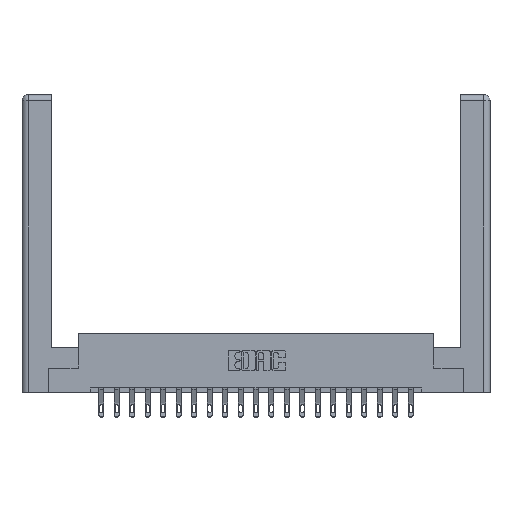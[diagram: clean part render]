
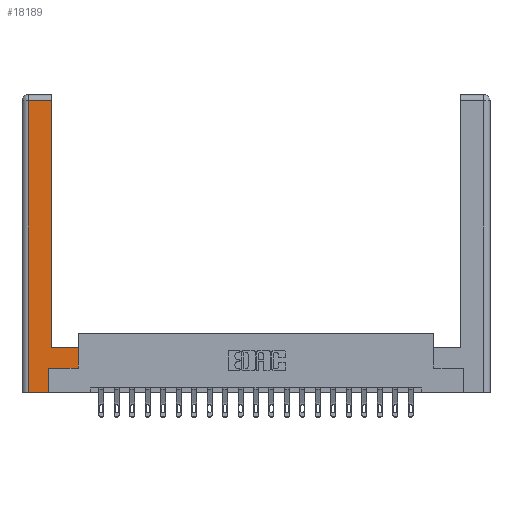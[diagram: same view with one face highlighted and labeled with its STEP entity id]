
A CAD part, top view. The second image highlights one B-rep face of the part: STEP entity #18189.
In plain terms, the highlighted planar face has unit normal (0, 0, 1).
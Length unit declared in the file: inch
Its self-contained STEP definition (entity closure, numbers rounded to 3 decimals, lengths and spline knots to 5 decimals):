
#303 = EDGE_CURVE ( 'NONE', #4934, #14037, #21726, .T. ) ;
#592 = VERTEX_POINT ( 'NONE', #5623 ) ;
#604 = DIRECTION ( 'NONE',  ( 1., 0., 0. ) ) ;
#1045 = CARTESIAN_POINT ( 'NONE',  ( 0.0615, 0., 0. ) ) ;
#1606 = DIRECTION ( 'NONE',  ( 1., 0., 0. ) ) ;
#1662 = LINE ( 'NONE', #15272, #3264 ) ;
#2182 = VECTOR ( 'NONE', #604, 39.37008 ) ;
#2737 = DIRECTION ( 'NONE',  ( -1., 0., 0. ) ) ;
#2754 = ORIENTED_EDGE ( 'NONE', *, *, #4813, .T. ) ;
#2914 = EDGE_LOOP ( 'NONE', ( #16398, #19296, #11142, #20492, #2754, #13698, #19203, #19072 ) ) ;
#3264 = VECTOR ( 'NONE', #1606, 39.37008 ) ;
#3643 = DIRECTION ( 'NONE',  ( 0., 1., 0. ) ) ;
#3861 = LINE ( 'NONE', #11119, #15807 ) ;
#4012 = LINE ( 'NONE', #9104, #15720 ) ;
#4514 = CARTESIAN_POINT ( 'NONE',  ( 0.565, 0.45, 0. ) ) ;
#4813 = EDGE_CURVE ( 'NONE', #12583, #592, #6343, .T. ) ;
#4861 = CARTESIAN_POINT ( 'NONE',  ( 0.265, 0., 0. ) ) ;
#4934 = VERTEX_POINT ( 'NONE', #6901 ) ;
#5126 = DIRECTION ( 'NONE',  ( 0., 0., -1. ) ) ;
#5623 = CARTESIAN_POINT ( 'NONE',  ( 0.265, 0.245, 0. ) ) ;
#5866 = CARTESIAN_POINT ( 'NONE',  ( 0.0615, 0., 0. ) ) ;
#5946 = DIRECTION ( 'NONE',  ( 0., -1., 0. ) ) ;
#6016 = CARTESIAN_POINT ( 'NONE',  ( 0.295, 2.94, 0. ) ) ;
#6152 = EDGE_CURVE ( 'NONE', #15660, #20231, #3861, .T. ) ;
#6343 = LINE ( 'NONE', #16733, #9555 ) ;
#6764 = CARTESIAN_POINT ( 'NONE',  ( 0., 0., 0. ) ) ;
#6901 = CARTESIAN_POINT ( 'NONE',  ( 0.0615, 2.94, 0. ) ) ;
#7133 = CARTESIAN_POINT ( 'NONE',  ( 0.295, 3., 0. ) ) ;
#7845 = LINE ( 'NONE', #7133, #21127 ) ;
#8257 = EDGE_CURVE ( 'NONE', #592, #13716, #12026, .T. ) ;
#9019 = CARTESIAN_POINT ( 'NONE',  ( 0.565, 0.245, 0. ) ) ;
#9048 = EDGE_CURVE ( 'NONE', #20231, #12795, #7845, .T. ) ;
#9104 = CARTESIAN_POINT ( 'NONE',  ( 0.0615, 2.94, 0. ) ) ;
#9362 = VECTOR ( 'NONE', #16579, 39.37008 ) ;
#9555 = VECTOR ( 'NONE', #11904, 39.37008 ) ;
#9833 = CARTESIAN_POINT ( 'NONE',  ( 0.565, 0.45, 0. ) ) ;
#10661 = DIRECTION ( 'NONE',  ( -1., 0., 0. ) ) ;
#11119 = CARTESIAN_POINT ( 'NONE',  ( 0.295, 0.45, 0. ) ) ;
#11142 = ORIENTED_EDGE ( 'NONE', *, *, #303, .T. ) ;
#11904 = DIRECTION ( 'NONE',  ( 0., 1., 0. ) ) ;
#12026 = LINE ( 'NONE', #9019, #2182 ) ;
#12583 = VERTEX_POINT ( 'NONE', #4861 ) ;
#12795 = VERTEX_POINT ( 'NONE', #6016 ) ;
#13532 = PLANE ( 'NONE',  #14444 ) ;
#13646 = EDGE_CURVE ( 'NONE', #14037, #12583, #1662, .T. ) ;
#13698 = ORIENTED_EDGE ( 'NONE', *, *, #8257, .T. ) ;
#13716 = VERTEX_POINT ( 'NONE', #18994 ) ;
#13880 = LINE ( 'NONE', #9833, #9362 ) ;
#14037 = VERTEX_POINT ( 'NONE', #1045 ) ;
#14373 = CARTESIAN_POINT ( 'NONE',  ( 0.295, 0.45, 0. ) ) ;
#14444 = AXIS2_PLACEMENT_3D ( 'NONE', #6764, #5126, #20420 ) ;
#14504 = EDGE_CURVE ( 'NONE', #13716, #15660, #13880, .T. ) ;
#14823 = VECTOR ( 'NONE', #5946, 39.37008 ) ;
#15272 = CARTESIAN_POINT ( 'NONE',  ( 0.265, 0., 0. ) ) ;
#15660 = VERTEX_POINT ( 'NONE', #4514 ) ;
#15720 = VECTOR ( 'NONE', #10661, 39.37008 ) ;
#15807 = VECTOR ( 'NONE', #2737, 39.37008 ) ;
#16398 = ORIENTED_EDGE ( 'NONE', *, *, #9048, .T. ) ;
#16579 = DIRECTION ( 'NONE',  ( 0., 1., 0. ) ) ;
#16733 = CARTESIAN_POINT ( 'NONE',  ( 0.265, 0.245, 0. ) ) ;
#18189 = ADVANCED_FACE ( 'NONE', ( #19513 ), #13532, .F. ) ;
#18994 = CARTESIAN_POINT ( 'NONE',  ( 0.565, 0.245, 0. ) ) ;
#19072 = ORIENTED_EDGE ( 'NONE', *, *, #6152, .T. ) ;
#19203 = ORIENTED_EDGE ( 'NONE', *, *, #14504, .T. ) ;
#19296 = ORIENTED_EDGE ( 'NONE', *, *, #20478, .T. ) ;
#19513 = FACE_OUTER_BOUND ( 'NONE', #2914, .T. ) ;
#20231 = VERTEX_POINT ( 'NONE', #14373 ) ;
#20420 = DIRECTION ( 'NONE',  ( -1., 0., 0. ) ) ;
#20478 = EDGE_CURVE ( 'NONE', #12795, #4934, #4012, .T. ) ;
#20492 = ORIENTED_EDGE ( 'NONE', *, *, #13646, .T. ) ;
#21127 = VECTOR ( 'NONE', #3643, 39.37008 ) ;
#21726 = LINE ( 'NONE', #5866, #14823 ) ;
